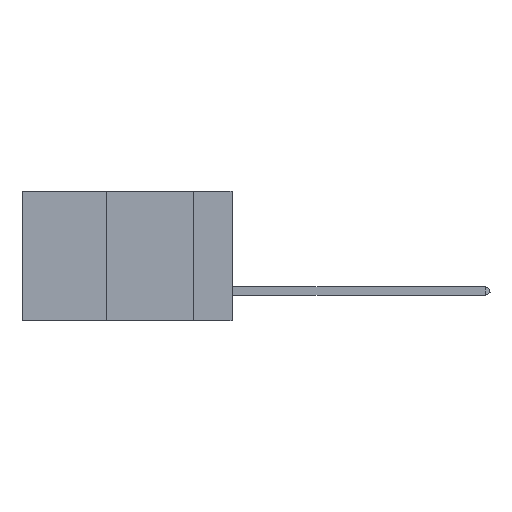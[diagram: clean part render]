
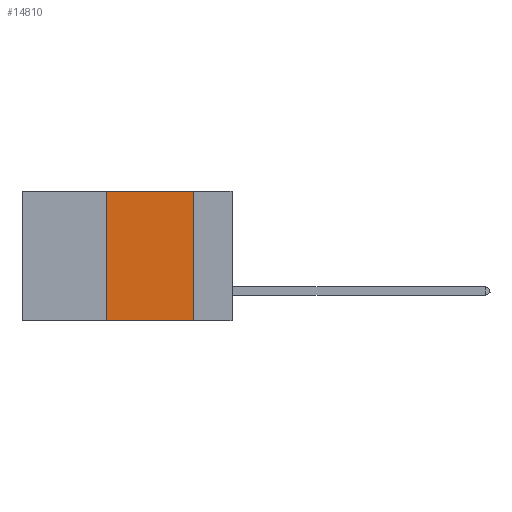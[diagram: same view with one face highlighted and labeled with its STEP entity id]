
A CAD part, left-side view. The second image highlights one B-rep face of the part: STEP entity #14810.
In plain terms, the highlighted planar face has unit normal (-1, 0, 0).
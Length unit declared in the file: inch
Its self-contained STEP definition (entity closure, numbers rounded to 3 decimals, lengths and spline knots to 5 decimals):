
#162 = DIRECTION ( 'NONE',  ( 0., 0., -1. ) ) ;
#790 = EDGE_CURVE ( 'NONE', #7119, #17936, #29911, .T. ) ;
#5604 = CARTESIAN_POINT ( 'NONE',  ( 0., 0.6, 0. ) ) ;
#5656 = FACE_OUTER_BOUND ( 'NONE', #24702, .T. ) ;
#5702 = DIRECTION ( 'NONE',  ( 0., 0., -1. ) ) ;
#5810 = LINE ( 'NONE', #7341, #19476 ) ;
#7119 = VERTEX_POINT ( 'NONE', #16933 ) ;
#7341 = CARTESIAN_POINT ( 'NONE',  ( 0., 0.11, 0. ) ) ;
#8131 = DIRECTION ( 'NONE',  ( 0., -1., 0. ) ) ;
#9275 = ORIENTED_EDGE ( 'NONE', *, *, #12055, .F. ) ;
#10485 = DIRECTION ( 'NONE',  ( 0., 0., 1. ) ) ;
#10665 = CARTESIAN_POINT ( 'NONE',  ( 0., 0.6, -0.37 ) ) ;
#10984 = VERTEX_POINT ( 'NONE', #21844 ) ;
#12055 = EDGE_CURVE ( 'NONE', #10984, #17936, #5810, .T. ) ;
#13064 = VECTOR ( 'NONE', #32244, 39.37008 ) ;
#14810 = ADVANCED_FACE ( 'NONE', ( #5656 ), #21411, .F. ) ;
#15331 = ORIENTED_EDGE ( 'NONE', *, *, #24964, .F. ) ;
#15461 = CARTESIAN_POINT ( 'NONE',  ( 0., 0.36, 0. ) ) ;
#16933 = CARTESIAN_POINT ( 'NONE',  ( 0., 0.36, -0.37 ) ) ;
#17271 = VECTOR ( 'NONE', #10485, 39.37008 ) ;
#17936 = VERTEX_POINT ( 'NONE', #22857 ) ;
#19476 = VECTOR ( 'NONE', #5702, 39.37008 ) ;
#19765 = VERTEX_POINT ( 'NONE', #25330 ) ;
#21411 = PLANE ( 'NONE',  #31626 ) ;
#21844 = CARTESIAN_POINT ( 'NONE',  ( 0., 0.11, 0. ) ) ;
#22631 = LINE ( 'NONE', #24247, #13064 ) ;
#22857 = CARTESIAN_POINT ( 'NONE',  ( 0., 0.11, -0.37 ) ) ;
#23047 = ORIENTED_EDGE ( 'NONE', *, *, #26229, .F. ) ;
#24085 = VECTOR ( 'NONE', #8131, 39.37008 ) ;
#24247 = CARTESIAN_POINT ( 'NONE',  ( 0., 0.6, 0. ) ) ;
#24272 = LINE ( 'NONE', #15461, #17271 ) ;
#24702 = EDGE_LOOP ( 'NONE', ( #9275, #23047, #15331, #25273 ) ) ;
#24964 = EDGE_CURVE ( 'NONE', #7119, #19765, #24272, .T. ) ;
#25273 = ORIENTED_EDGE ( 'NONE', *, *, #790, .T. ) ;
#25330 = CARTESIAN_POINT ( 'NONE',  ( 0., 0.36, 0. ) ) ;
#26229 = EDGE_CURVE ( 'NONE', #19765, #10984, #22631, .T. ) ;
#29911 = LINE ( 'NONE', #10665, #24085 ) ;
#31626 = AXIS2_PLACEMENT_3D ( 'NONE', #5604, #31955, #162 ) ;
#31955 = DIRECTION ( 'NONE',  ( 1., 0., 0. ) ) ;
#32244 = DIRECTION ( 'NONE',  ( 0., -1., 0. ) ) ;
